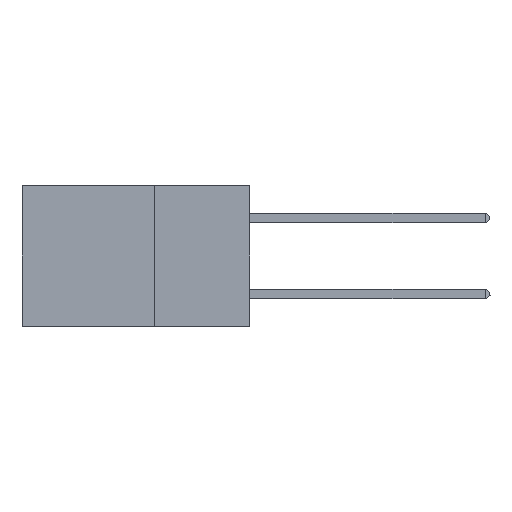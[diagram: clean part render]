
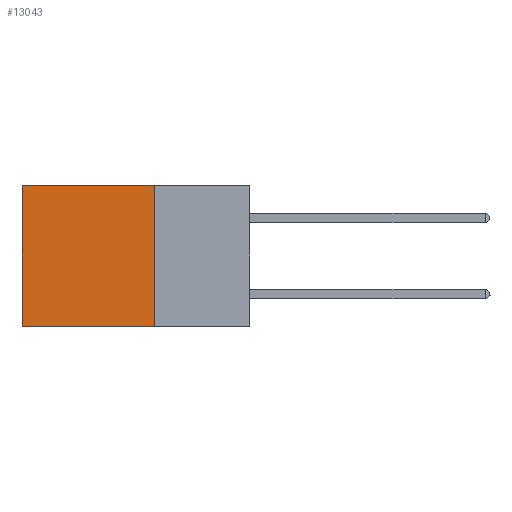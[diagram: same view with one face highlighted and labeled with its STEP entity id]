
A CAD part, left-side view. The second image highlights one B-rep face of the part: STEP entity #13043.
In plain terms, the highlighted planar face has unit normal (-1, 0, 0).
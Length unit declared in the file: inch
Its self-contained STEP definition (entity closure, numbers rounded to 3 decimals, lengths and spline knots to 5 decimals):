
#404 = EDGE_CURVE ( 'NONE', #1079, #13380, #8680, .T. ) ;
#552 = CARTESIAN_POINT ( 'NONE',  ( 0.2875, 0.25, 0. ) ) ;
#1079 = VERTEX_POINT ( 'NONE', #3799 ) ;
#1553 = DIRECTION ( 'NONE',  ( 0., 0., -1. ) ) ;
#1979 = CARTESIAN_POINT ( 'NONE',  ( 0.2875, 0.25, 0. ) ) ;
#3282 = CARTESIAN_POINT ( 'NONE',  ( 0.2875, 0.25, 0. ) ) ;
#3799 = CARTESIAN_POINT ( 'NONE',  ( 0.2875, 0.6, 0. ) ) ;
#4914 = VECTOR ( 'NONE', #16581, 39.37008 ) ;
#5397 = EDGE_CURVE ( 'NONE', #20719, #1079, #20842, .T. ) ;
#5687 = FACE_OUTER_BOUND ( 'NONE', #25935, .T. ) ;
#7573 = CARTESIAN_POINT ( 'NONE',  ( 0.2875, 0.25, -0.37 ) ) ;
#7584 = DIRECTION ( 'NONE',  ( 0., 1., 0. ) ) ;
#8680 = LINE ( 'NONE', #14124, #18791 ) ;
#12826 = PLANE ( 'NONE',  #16481 ) ;
#13043 = ADVANCED_FACE ( 'NONE', ( #5687 ), #12826, .F. ) ;
#13380 = VERTEX_POINT ( 'NONE', #20172 ) ;
#13926 = LINE ( 'NONE', #26783, #20779 ) ;
#14124 = CARTESIAN_POINT ( 'NONE',  ( 0.2875, 0.6, 0. ) ) ;
#15698 = CARTESIAN_POINT ( 'NONE',  ( 0.2875, 0.25, 0. ) ) ;
#16481 = AXIS2_PLACEMENT_3D ( 'NONE', #552, #23450, #19060 ) ;
#16581 = DIRECTION ( 'NONE',  ( 0., 0., -1. ) ) ;
#18791 = VECTOR ( 'NONE', #1553, 39.37008 ) ;
#19060 = DIRECTION ( 'NONE',  ( 0., 0., -1. ) ) ;
#19691 = VERTEX_POINT ( 'NONE', #7573 ) ;
#19976 = ORIENTED_EDGE ( 'NONE', *, *, #25701, .F. ) ;
#20172 = CARTESIAN_POINT ( 'NONE',  ( 0.2875, 0.6, -0.37 ) ) ;
#20719 = VERTEX_POINT ( 'NONE', #3282 ) ;
#20779 = VECTOR ( 'NONE', #22516, 39.37008 ) ;
#20842 = LINE ( 'NONE', #15698, #26083 ) ;
#21374 = ORIENTED_EDGE ( 'NONE', *, *, #5397, .T. ) ;
#22516 = DIRECTION ( 'NONE',  ( 0., 1., 0. ) ) ;
#22952 = EDGE_CURVE ( 'NONE', #20719, #19691, #25492, .T. ) ;
#23450 = DIRECTION ( 'NONE',  ( 1., 0., 0. ) ) ;
#23801 = ORIENTED_EDGE ( 'NONE', *, *, #404, .T. ) ;
#25492 = LINE ( 'NONE', #1979, #4914 ) ;
#25701 = EDGE_CURVE ( 'NONE', #19691, #13380, #13926, .T. ) ;
#25935 = EDGE_LOOP ( 'NONE', ( #23801, #19976, #26610, #21374 ) ) ;
#26083 = VECTOR ( 'NONE', #7584, 39.37008 ) ;
#26610 = ORIENTED_EDGE ( 'NONE', *, *, #22952, .F. ) ;
#26783 = CARTESIAN_POINT ( 'NONE',  ( 0.2875, 0.25, -0.37 ) ) ;
